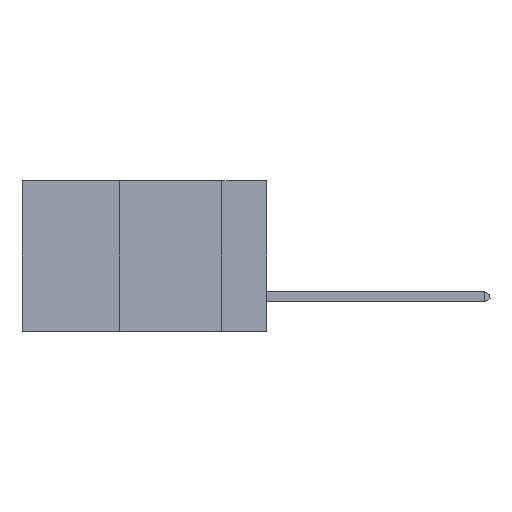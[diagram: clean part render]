
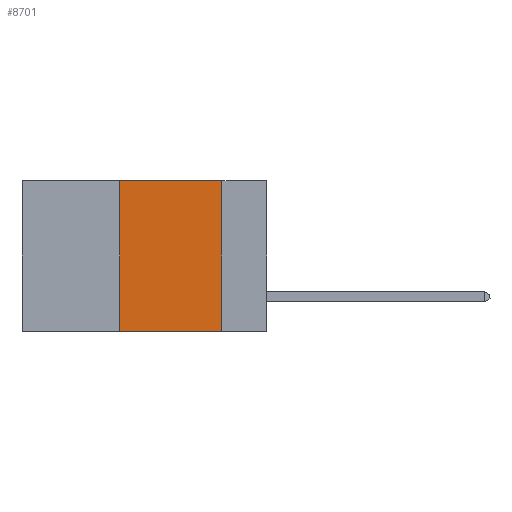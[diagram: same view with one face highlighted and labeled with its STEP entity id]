
A CAD part, left-side view. The second image highlights one B-rep face of the part: STEP entity #8701.
In plain terms, the highlighted planar face has unit normal (-1, 0, 0).
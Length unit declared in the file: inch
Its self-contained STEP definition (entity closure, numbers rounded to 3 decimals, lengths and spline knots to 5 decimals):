
#529 = VECTOR ( 'NONE', #22461, 39.37008 ) ;
#615 = CARTESIAN_POINT ( 'NONE',  ( 0., 0.11, 0. ) ) ;
#1163 = CARTESIAN_POINT ( 'NONE',  ( 0., 0.6, -0.37 ) ) ;
#2514 = VERTEX_POINT ( 'NONE', #7712 ) ;
#2649 = VERTEX_POINT ( 'NONE', #8151 ) ;
#3070 = DIRECTION ( 'NONE',  ( 0., 0., -1. ) ) ;
#3270 = ORIENTED_EDGE ( 'NONE', *, *, #25046, .F. ) ;
#4327 = LINE ( 'NONE', #8599, #29264 ) ;
#7655 = LINE ( 'NONE', #1163, #529 ) ;
#7712 = CARTESIAN_POINT ( 'NONE',  ( 0., 0.36, -0.37 ) ) ;
#8151 = CARTESIAN_POINT ( 'NONE',  ( 0., 0.11, -0.37 ) ) ;
#8180 = CARTESIAN_POINT ( 'NONE',  ( 0., 0.11, 0. ) ) ;
#8599 = CARTESIAN_POINT ( 'NONE',  ( 0., 0.36, 0. ) ) ;
#8701 = ADVANCED_FACE ( 'NONE', ( #13978 ), #26250, .F. ) ;
#8997 = EDGE_CURVE ( 'NONE', #2514, #19580, #4327, .T. ) ;
#9931 = ORIENTED_EDGE ( 'NONE', *, *, #8997, .F. ) ;
#10002 = ORIENTED_EDGE ( 'NONE', *, *, #14346, .T. ) ;
#10242 = LINE ( 'NONE', #615, #28174 ) ;
#12231 = DIRECTION ( 'NONE',  ( 1., 0., 0. ) ) ;
#13978 = FACE_OUTER_BOUND ( 'NONE', #24280, .T. ) ;
#14302 = VERTEX_POINT ( 'NONE', #8180 ) ;
#14346 = EDGE_CURVE ( 'NONE', #2514, #2649, #7655, .T. ) ;
#16551 = VECTOR ( 'NONE', #24913, 39.37008 ) ;
#16898 = ORIENTED_EDGE ( 'NONE', *, *, #25526, .F. ) ;
#19218 = CARTESIAN_POINT ( 'NONE',  ( 0., 0.6, 0. ) ) ;
#19580 = VERTEX_POINT ( 'NONE', #22860 ) ;
#22461 = DIRECTION ( 'NONE',  ( 0., -1., 0. ) ) ;
#22695 = AXIS2_PLACEMENT_3D ( 'NONE', #19218, #12231, #28578 ) ;
#22744 = LINE ( 'NONE', #29470, #16551 ) ;
#22860 = CARTESIAN_POINT ( 'NONE',  ( 0., 0.36, 0. ) ) ;
#24280 = EDGE_LOOP ( 'NONE', ( #16898, #3270, #9931, #10002 ) ) ;
#24913 = DIRECTION ( 'NONE',  ( 0., -1., 0. ) ) ;
#25008 = DIRECTION ( 'NONE',  ( 0., 0., 1. ) ) ;
#25046 = EDGE_CURVE ( 'NONE', #19580, #14302, #22744, .T. ) ;
#25526 = EDGE_CURVE ( 'NONE', #14302, #2649, #10242, .T. ) ;
#26250 = PLANE ( 'NONE',  #22695 ) ;
#28174 = VECTOR ( 'NONE', #3070, 39.37008 ) ;
#28578 = DIRECTION ( 'NONE',  ( 0., 0., -1. ) ) ;
#29264 = VECTOR ( 'NONE', #25008, 39.37008 ) ;
#29470 = CARTESIAN_POINT ( 'NONE',  ( 0., 0.6, 0. ) ) ;
